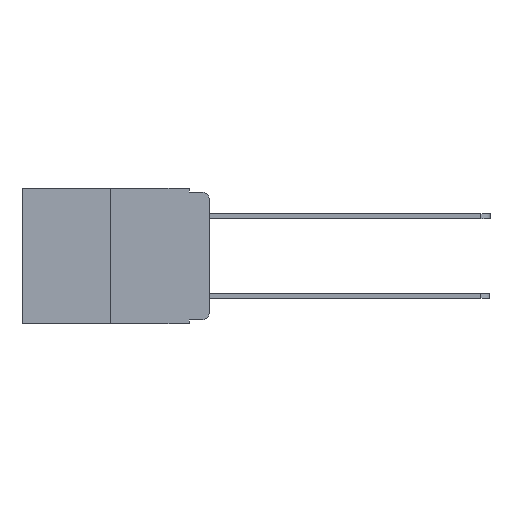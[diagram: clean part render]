
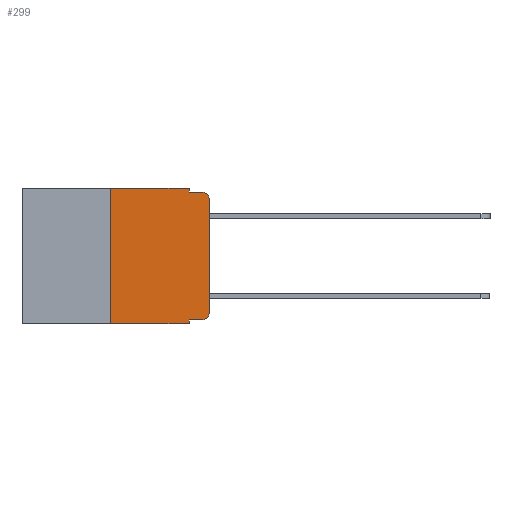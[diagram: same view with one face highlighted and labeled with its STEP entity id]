
A CAD part, left-side view. The second image highlights one B-rep face of the part: STEP entity #299.
In plain terms, the highlighted planar face has unit normal (-1, 0, 0).
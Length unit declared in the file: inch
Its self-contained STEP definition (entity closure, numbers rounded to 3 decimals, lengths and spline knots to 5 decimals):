
#225 = EDGE_CURVE ( 'NONE', #11789, #4591, #4919, .T. ) ;
#299 = ADVANCED_FACE ( 'NONE', ( #14104 ), #8979, .F. ) ;
#911 = ORIENTED_EDGE ( 'NONE', *, *, #225, .T. ) ;
#981 = AXIS2_PLACEMENT_3D ( 'NONE', #4659, #15183, #6237 ) ;
#1214 = VECTOR ( 'NONE', #18858, 39.37008 ) ;
#1486 = DIRECTION ( 'NONE',  ( 0., -1., 0. ) ) ;
#1600 = ORIENTED_EDGE ( 'NONE', *, *, #5274, .F. ) ;
#1645 = ORIENTED_EDGE ( 'NONE', *, *, #7332, .T. ) ;
#2156 = EDGE_LOOP ( 'NONE', ( #12585, #4055, #9567, #12957, #1600, #5826, #1645, #5820, #13660, #911 ) ) ;
#2641 = CARTESIAN_POINT ( 'NONE',  ( 0., 0.051, -0.333 ) ) ;
#2684 = VERTEX_POINT ( 'NONE', #10263 ) ;
#2708 = CARTESIAN_POINT ( 'NONE',  ( 0., 0.02, -0.313 ) ) ;
#3459 = CARTESIAN_POINT ( 'NONE',  ( 0., 0.25, 0. ) ) ;
#3766 = VECTOR ( 'NONE', #11279, 39.37008 ) ;
#4055 = ORIENTED_EDGE ( 'NONE', *, *, #11926, .T. ) ;
#4301 = DIRECTION ( 'NONE',  ( 0., 0., -1. ) ) ;
#4383 = VECTOR ( 'NONE', #5525, 39.37008 ) ;
#4591 = VERTEX_POINT ( 'NONE', #15625 ) ;
#4659 = CARTESIAN_POINT ( 'NONE',  ( 0., 0.02, -0.03 ) ) ;
#4795 = DIRECTION ( 'NONE',  ( 0., 0., -1. ) ) ;
#4847 = DIRECTION ( 'NONE',  ( -1., 0., 0. ) ) ;
#4861 = LINE ( 'NONE', #13023, #4383 ) ;
#4896 = EDGE_CURVE ( 'NONE', #11743, #15232, #11900, .T. ) ;
#4919 = CIRCLE ( 'NONE', #14812, 0.02 ) ;
#5011 = DIRECTION ( 'NONE',  ( 0., 0., 1. ) ) ;
#5274 = EDGE_CURVE ( 'NONE', #2684, #15888, #8356, .T. ) ;
#5308 = DIRECTION ( 'NONE',  ( 0., -1., 0. ) ) ;
#5384 = CARTESIAN_POINT ( 'NONE',  ( 0., 0.473, 0. ) ) ;
#5466 = LINE ( 'NONE', #8631, #1214 ) ;
#5519 = LINE ( 'NONE', #10794, #6001 ) ;
#5525 = DIRECTION ( 'NONE',  ( 0., -1., 0. ) ) ;
#5550 = LINE ( 'NONE', #3459, #9144 ) ;
#5820 = ORIENTED_EDGE ( 'NONE', *, *, #4896, .F. ) ;
#5826 = ORIENTED_EDGE ( 'NONE', *, *, #16289, .F. ) ;
#6001 = VECTOR ( 'NONE', #19557, 39.37008 ) ;
#6237 = DIRECTION ( 'NONE',  ( 0., 0., -1. ) ) ;
#7332 = EDGE_CURVE ( 'NONE', #12296, #15232, #4861, .T. ) ;
#7901 = VECTOR ( 'NONE', #4301, 39.37008 ) ;
#8356 = LINE ( 'NONE', #5384, #19658 ) ;
#8517 = CARTESIAN_POINT ( 'NONE',  ( 0., 0.051, -0.01 ) ) ;
#8631 = CARTESIAN_POINT ( 'NONE',  ( 0., 0.051, 0. ) ) ;
#8869 = CARTESIAN_POINT ( 'NONE',  ( 0., 0.051, 0. ) ) ;
#8979 = PLANE ( 'NONE',  #17370 ) ;
#9048 = CARTESIAN_POINT ( 'NONE',  ( 0., 0.473, 0. ) ) ;
#9144 = VECTOR ( 'NONE', #5011, 39.37008 ) ;
#9567 = ORIENTED_EDGE ( 'NONE', *, *, #11497, .F. ) ;
#9651 = VERTEX_POINT ( 'NONE', #8517 ) ;
#9807 = CARTESIAN_POINT ( 'NONE',  ( 0., 0.051, -0.01 ) ) ;
#10263 = CARTESIAN_POINT ( 'NONE',  ( 0., 0.25, 0. ) ) ;
#10737 = EDGE_CURVE ( 'NONE', #4591, #11144, #5519, .T. ) ;
#10794 = CARTESIAN_POINT ( 'NONE',  ( 0., 0., 0. ) ) ;
#11144 = VERTEX_POINT ( 'NONE', #12019 ) ;
#11279 = DIRECTION ( 'NONE',  ( 0., -1., 0. ) ) ;
#11284 = EDGE_CURVE ( 'NONE', #11743, #11789, #16470, .T. ) ;
#11497 = EDGE_CURVE ( 'NONE', #9651, #16560, #19656, .T. ) ;
#11743 = VERTEX_POINT ( 'NONE', #2641 ) ;
#11789 = VERTEX_POINT ( 'NONE', #14862 ) ;
#11822 = CARTESIAN_POINT ( 'NONE',  ( 0., 0.051, 0. ) ) ;
#11900 = LINE ( 'NONE', #11822, #7901 ) ;
#11926 = EDGE_CURVE ( 'NONE', #11144, #16560, #12779, .T. ) ;
#12019 = CARTESIAN_POINT ( 'NONE',  ( 0., 0., -0.03 ) ) ;
#12124 = VECTOR ( 'NONE', #1486, 39.37008 ) ;
#12296 = VERTEX_POINT ( 'NONE', #13062 ) ;
#12384 = EDGE_CURVE ( 'NONE', #15888, #9651, #5466, .T. ) ;
#12585 = ORIENTED_EDGE ( 'NONE', *, *, #10737, .T. ) ;
#12779 = CIRCLE ( 'NONE', #981, 0.02 ) ;
#12957 = ORIENTED_EDGE ( 'NONE', *, *, #12384, .F. ) ;
#13023 = CARTESIAN_POINT ( 'NONE',  ( 0., 0.473, -0.343 ) ) ;
#13062 = CARTESIAN_POINT ( 'NONE',  ( 0., 0.25, -0.343 ) ) ;
#13660 = ORIENTED_EDGE ( 'NONE', *, *, #11284, .T. ) ;
#14104 = FACE_OUTER_BOUND ( 'NONE', #2156, .T. ) ;
#14812 = AXIS2_PLACEMENT_3D ( 'NONE', #2708, #4847, #4795 ) ;
#14862 = CARTESIAN_POINT ( 'NONE',  ( 0., 0.02, -0.333 ) ) ;
#15183 = DIRECTION ( 'NONE',  ( -1., 0., 0. ) ) ;
#15232 = VERTEX_POINT ( 'NONE', #18894 ) ;
#15625 = CARTESIAN_POINT ( 'NONE',  ( 0., 0., -0.313 ) ) ;
#15888 = VERTEX_POINT ( 'NONE', #8869 ) ;
#16289 = EDGE_CURVE ( 'NONE', #12296, #2684, #5550, .T. ) ;
#16470 = LINE ( 'NONE', #18067, #12124 ) ;
#16560 = VERTEX_POINT ( 'NONE', #19062 ) ;
#17370 = AXIS2_PLACEMENT_3D ( 'NONE', #9048, #17806, #17718 ) ;
#17718 = DIRECTION ( 'NONE',  ( 0., 0., -1. ) ) ;
#17806 = DIRECTION ( 'NONE',  ( 1., 0., 0. ) ) ;
#18067 = CARTESIAN_POINT ( 'NONE',  ( 0., 0.051, -0.333 ) ) ;
#18858 = DIRECTION ( 'NONE',  ( 0., 0., -1. ) ) ;
#18894 = CARTESIAN_POINT ( 'NONE',  ( 0., 0.051, -0.343 ) ) ;
#19062 = CARTESIAN_POINT ( 'NONE',  ( 0., 0.02, -0.01 ) ) ;
#19557 = DIRECTION ( 'NONE',  ( 0., 0., 1. ) ) ;
#19656 = LINE ( 'NONE', #9807, #3766 ) ;
#19658 = VECTOR ( 'NONE', #5308, 39.37008 ) ;
